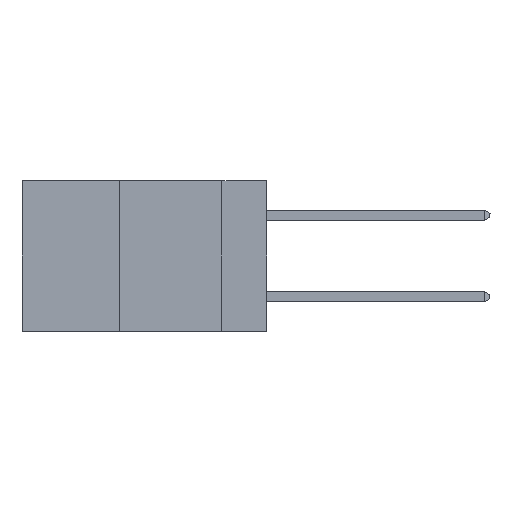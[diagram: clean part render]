
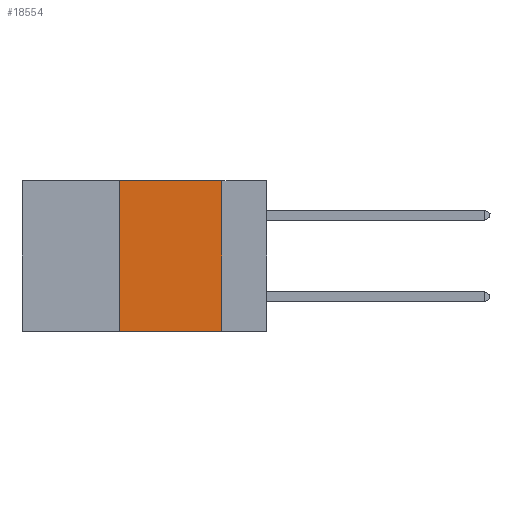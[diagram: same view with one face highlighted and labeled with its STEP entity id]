
A CAD part, left-side view. The second image highlights one B-rep face of the part: STEP entity #18554.
In plain terms, the highlighted planar face has unit normal (-1, 0, 0).
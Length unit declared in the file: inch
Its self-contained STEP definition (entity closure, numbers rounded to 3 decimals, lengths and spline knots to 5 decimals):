
#544 = CARTESIAN_POINT ( 'NONE',  ( 0., 0.36, 0. ) ) ;
#716 = AXIS2_PLACEMENT_3D ( 'NONE', #19777, #4734, #9493 ) ;
#1062 = DIRECTION ( 'NONE',  ( 0., 0., 1. ) ) ;
#1307 = PLANE ( 'NONE',  #716 ) ;
#2248 = CARTESIAN_POINT ( 'NONE',  ( 0., 0.36, -0.37 ) ) ;
#2848 = FACE_OUTER_BOUND ( 'NONE', #7217, .T. ) ;
#4734 = DIRECTION ( 'NONE',  ( 1., 0., 0. ) ) ;
#5234 = VECTOR ( 'NONE', #1062, 39.37008 ) ;
#5342 = LINE ( 'NONE', #10769, #16790 ) ;
#5798 = CARTESIAN_POINT ( 'NONE',  ( 0., 0.11, 0. ) ) ;
#6454 = DIRECTION ( 'NONE',  ( 0., 0., -1. ) ) ;
#7217 = EDGE_LOOP ( 'NONE', ( #19186, #15404, #7325, #13620 ) ) ;
#7325 = ORIENTED_EDGE ( 'NONE', *, *, #18954, .F. ) ;
#8019 = LINE ( 'NONE', #17983, #5234 ) ;
#8333 = EDGE_CURVE ( 'NONE', #9061, #16130, #17957, .T. ) ;
#8380 = EDGE_CURVE ( 'NONE', #16130, #10722, #10305, .T. ) ;
#9061 = VERTEX_POINT ( 'NONE', #544 ) ;
#9493 = DIRECTION ( 'NONE',  ( 0., 0., -1. ) ) ;
#9891 = CARTESIAN_POINT ( 'NONE',  ( 0., 0.11, 0. ) ) ;
#10042 = EDGE_CURVE ( 'NONE', #10058, #10722, #5342, .T. ) ;
#10058 = VERTEX_POINT ( 'NONE', #2248 ) ;
#10305 = LINE ( 'NONE', #9891, #11399 ) ;
#10722 = VERTEX_POINT ( 'NONE', #16883 ) ;
#10769 = CARTESIAN_POINT ( 'NONE',  ( 0., 0.6, -0.37 ) ) ;
#11399 = VECTOR ( 'NONE', #6454, 39.37008 ) ;
#12106 = DIRECTION ( 'NONE',  ( 0., -1., 0. ) ) ;
#13620 = ORIENTED_EDGE ( 'NONE', *, *, #10042, .T. ) ;
#15404 = ORIENTED_EDGE ( 'NONE', *, *, #8333, .F. ) ;
#16130 = VERTEX_POINT ( 'NONE', #5798 ) ;
#16790 = VECTOR ( 'NONE', #12106, 39.37008 ) ;
#16883 = CARTESIAN_POINT ( 'NONE',  ( 0., 0.11, -0.37 ) ) ;
#17957 = LINE ( 'NONE', #19400, #18117 ) ;
#17983 = CARTESIAN_POINT ( 'NONE',  ( 0., 0.36, 0. ) ) ;
#18117 = VECTOR ( 'NONE', #20969, 39.37008 ) ;
#18554 = ADVANCED_FACE ( 'NONE', ( #2848 ), #1307, .F. ) ;
#18954 = EDGE_CURVE ( 'NONE', #10058, #9061, #8019, .T. ) ;
#19186 = ORIENTED_EDGE ( 'NONE', *, *, #8380, .F. ) ;
#19400 = CARTESIAN_POINT ( 'NONE',  ( 0., 0.6, 0. ) ) ;
#19777 = CARTESIAN_POINT ( 'NONE',  ( 0., 0.6, 0. ) ) ;
#20969 = DIRECTION ( 'NONE',  ( 0., -1., 0. ) ) ;
